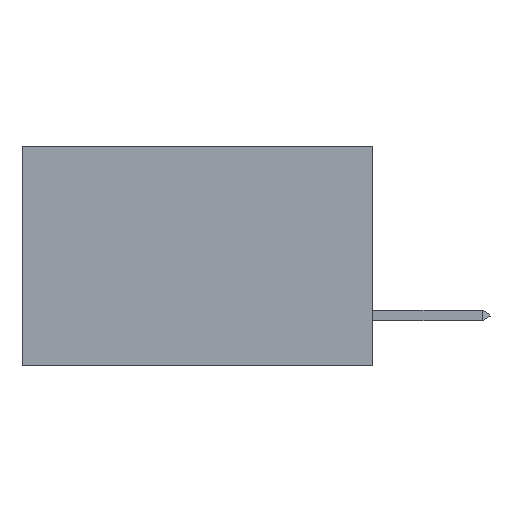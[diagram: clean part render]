
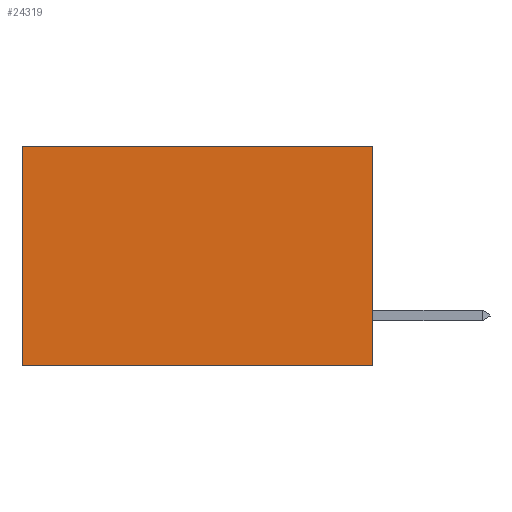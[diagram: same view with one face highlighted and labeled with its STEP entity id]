
A CAD part, left-side view. The second image highlights one B-rep face of the part: STEP entity #24319.
In plain terms, the highlighted planar face has unit normal (-1, 0, 0).
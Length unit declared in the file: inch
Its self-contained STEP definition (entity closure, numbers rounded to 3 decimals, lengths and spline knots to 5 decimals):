
#1491 = LINE ( 'NONE', #16703, #16572 ) ;
#2295 = CARTESIAN_POINT ( 'NONE',  ( 0.277, 0.59, 0. ) ) ;
#2305 = ORIENTED_EDGE ( 'NONE', *, *, #6828, .F. ) ;
#4025 = VECTOR ( 'NONE', #23313, 39.37008 ) ;
#4513 = EDGE_CURVE ( 'NONE', #16370, #10397, #6190, .T. ) ;
#4923 = ORIENTED_EDGE ( 'NONE', *, *, #13198, .F. ) ;
#6183 = PLANE ( 'NONE',  #21210 ) ;
#6190 = LINE ( 'NONE', #12197, #16889 ) ;
#6584 = CARTESIAN_POINT ( 'NONE',  ( 0.277, 0.59, -0.37 ) ) ;
#6828 = EDGE_CURVE ( 'NONE', #16370, #22783, #15166, .T. ) ;
#8346 = CARTESIAN_POINT ( 'NONE',  ( 0.277, 0., -0.37 ) ) ;
#8644 = EDGE_CURVE ( 'NONE', #10397, #19400, #15476, .T. ) ;
#8724 = DIRECTION ( 'NONE',  ( 0., 1., 0. ) ) ;
#10291 = ORIENTED_EDGE ( 'NONE', *, *, #4513, .T. ) ;
#10397 = VERTEX_POINT ( 'NONE', #2295 ) ;
#10504 = DIRECTION ( 'NONE',  ( 1., 0., 0. ) ) ;
#12197 = CARTESIAN_POINT ( 'NONE',  ( 0.277, 0., 0. ) ) ;
#12684 = CARTESIAN_POINT ( 'NONE',  ( 0.277, 0., -0.37 ) ) ;
#12709 = ORIENTED_EDGE ( 'NONE', *, *, #8644, .T. ) ;
#13198 = EDGE_CURVE ( 'NONE', #22783, #19400, #1491, .T. ) ;
#14513 = VECTOR ( 'NONE', #20230, 39.37008 ) ;
#14689 = DIRECTION ( 'NONE',  ( 0., 1., 0. ) ) ;
#15166 = LINE ( 'NONE', #20976, #14513 ) ;
#15243 = CARTESIAN_POINT ( 'NONE',  ( 0.277, 0., 0. ) ) ;
#15476 = LINE ( 'NONE', #23222, #4025 ) ;
#16370 = VERTEX_POINT ( 'NONE', #15243 ) ;
#16572 = VECTOR ( 'NONE', #14689, 39.37008 ) ;
#16703 = CARTESIAN_POINT ( 'NONE',  ( 0.277, 0., -0.37 ) ) ;
#16889 = VECTOR ( 'NONE', #8724, 39.37008 ) ;
#19400 = VERTEX_POINT ( 'NONE', #6584 ) ;
#19736 = EDGE_LOOP ( 'NONE', ( #12709, #4923, #2305, #10291 ) ) ;
#20230 = DIRECTION ( 'NONE',  ( 0., 0., -1. ) ) ;
#20976 = CARTESIAN_POINT ( 'NONE',  ( 0.277, 0., -0.37 ) ) ;
#21210 = AXIS2_PLACEMENT_3D ( 'NONE', #8346, #10504, #25080 ) ;
#22783 = VERTEX_POINT ( 'NONE', #12684 ) ;
#23222 = CARTESIAN_POINT ( 'NONE',  ( 0.277, 0.59, -0.37 ) ) ;
#23313 = DIRECTION ( 'NONE',  ( 0., 0., -1. ) ) ;
#24319 = ADVANCED_FACE ( 'NONE', ( #27212 ), #6183, .F. ) ;
#25080 = DIRECTION ( 'NONE',  ( 0., 0., -1. ) ) ;
#27212 = FACE_OUTER_BOUND ( 'NONE', #19736, .T. ) ;
